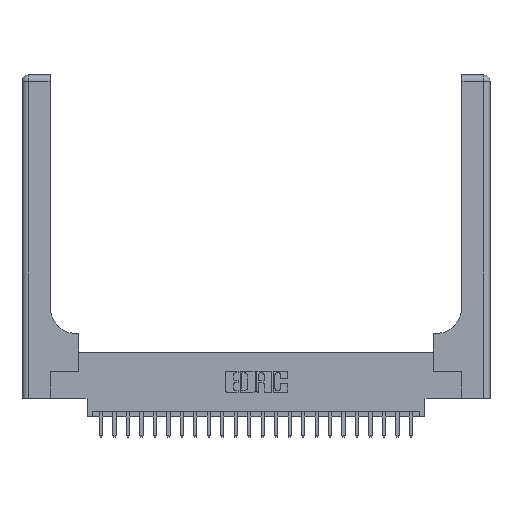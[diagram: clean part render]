
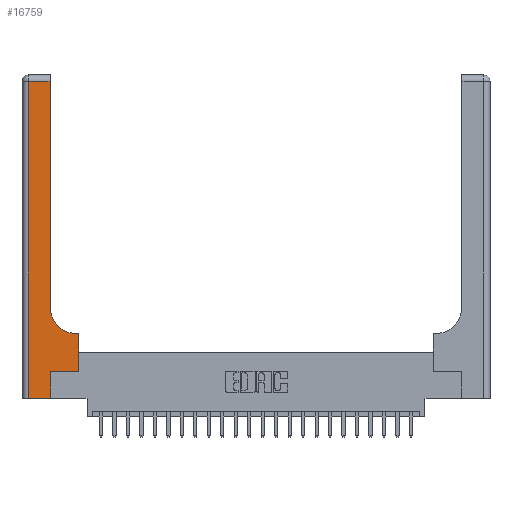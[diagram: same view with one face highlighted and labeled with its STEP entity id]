
A CAD part, top view. The second image highlights one B-rep face of the part: STEP entity #16759.
In plain terms, the highlighted planar face has unit normal (0, 0, 1).
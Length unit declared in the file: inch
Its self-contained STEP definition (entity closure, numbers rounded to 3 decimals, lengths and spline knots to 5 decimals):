
#467 = CARTESIAN_POINT ( 'NONE',  ( 0., 2.94, 0.37 ) ) ;
#500 = LINE ( 'NONE', #467, #5388 ) ;
#622 = ORIENTED_EDGE ( 'NONE', *, *, #14773, .T. ) ;
#769 = ORIENTED_EDGE ( 'NONE', *, *, #4746, .T. ) ;
#818 = EDGE_CURVE ( 'NONE', #1839, #12456, #20458, .T. ) ;
#1067 = ORIENTED_EDGE ( 'NONE', *, *, #16977, .T. ) ;
#1117 = AXIS2_PLACEMENT_3D ( 'NONE', #13332, #2342, #15140 ) ;
#1308 = ORIENTED_EDGE ( 'NONE', *, *, #20596, .T. ) ;
#1333 = CIRCLE ( 'NONE', #12049, 0.25 ) ;
#1466 = VERTEX_POINT ( 'NONE', #3202 ) ;
#1839 = VERTEX_POINT ( 'NONE', #16071 ) ;
#2086 = VERTEX_POINT ( 'NONE', #6284 ) ;
#2342 = DIRECTION ( 'NONE',  ( 0., 0., -1. ) ) ;
#2741 = CARTESIAN_POINT ( 'NONE',  ( 0.265, 0.25, 0.37 ) ) ;
#3039 = DIRECTION ( 'NONE',  ( -1., 0., 0. ) ) ;
#3202 = CARTESIAN_POINT ( 'NONE',  ( 0.26, 2.94, 0.37 ) ) ;
#3230 = EDGE_CURVE ( 'NONE', #19356, #1466, #9564, .T. ) ;
#4069 = VECTOR ( 'NONE', #13225, 39.37008 ) ;
#4310 = EDGE_CURVE ( 'NONE', #14408, #1839, #9453, .T. ) ;
#4746 = EDGE_CURVE ( 'NONE', #2086, #14117, #14071, .T. ) ;
#4954 = CARTESIAN_POINT ( 'NONE',  ( 0.26, 0.6, 0.37 ) ) ;
#5369 = ORIENTED_EDGE ( 'NONE', *, *, #3230, .T. ) ;
#5388 = VECTOR ( 'NONE', #11309, 39.37008 ) ;
#5515 = ORIENTED_EDGE ( 'NONE', *, *, #13615, .T. ) ;
#5915 = CARTESIAN_POINT ( 'NONE',  ( 0.26, 0.85, 0.37 ) ) ;
#6284 = CARTESIAN_POINT ( 'NONE',  ( 0.528, 0.25, 0.37 ) ) ;
#6522 = VECTOR ( 'NONE', #14974, 39.37008 ) ;
#7276 = LINE ( 'NONE', #4954, #16420 ) ;
#7803 = DIRECTION ( 'NONE',  ( 0., 0., -1. ) ) ;
#8040 = ORIENTED_EDGE ( 'NONE', *, *, #4310, .T. ) ;
#8920 = LINE ( 'NONE', #9505, #4069 ) ;
#9183 = VECTOR ( 'NONE', #17387, 39.37008 ) ;
#9430 = DIRECTION ( 'NONE',  ( 0., 1., 0. ) ) ;
#9453 = LINE ( 'NONE', #10834, #15457 ) ;
#9505 = CARTESIAN_POINT ( 'NONE',  ( 0.265, 0., 0.37 ) ) ;
#9511 = CARTESIAN_POINT ( 'NONE',  ( 0.26, 3., 0.37 ) ) ;
#9564 = LINE ( 'NONE', #9511, #18655 ) ;
#9961 = VERTEX_POINT ( 'NONE', #2741 ) ;
#10033 = CARTESIAN_POINT ( 'NONE',  ( 0.265, 0.25, 0.37 ) ) ;
#10834 = CARTESIAN_POINT ( 'NONE',  ( 0.06, 3., 0.37 ) ) ;
#10855 = VERTEX_POINT ( 'NONE', #13655 ) ;
#11309 = DIRECTION ( 'NONE',  ( -1., 0., 0. ) ) ;
#11474 = PLANE ( 'NONE',  #1117 ) ;
#11493 = CARTESIAN_POINT ( 'NONE',  ( 0.265, 0., 0.37 ) ) ;
#12049 = AXIS2_PLACEMENT_3D ( 'NONE', #18687, #7803, #20493 ) ;
#12456 = VERTEX_POINT ( 'NONE', #11493 ) ;
#13225 = DIRECTION ( 'NONE',  ( 0., 1., 0. ) ) ;
#13332 = CARTESIAN_POINT ( 'NONE',  ( 0., 3., 0.37 ) ) ;
#13438 = ORIENTED_EDGE ( 'NONE', *, *, #818, .T. ) ;
#13615 = EDGE_CURVE ( 'NONE', #1466, #14408, #500, .T. ) ;
#13655 = CARTESIAN_POINT ( 'NONE',  ( 0.51, 0.6, 0.37 ) ) ;
#14071 = LINE ( 'NONE', #19199, #9183 ) ;
#14117 = VERTEX_POINT ( 'NONE', #22760 ) ;
#14408 = VERTEX_POINT ( 'NONE', #18147 ) ;
#14773 = EDGE_CURVE ( 'NONE', #9961, #2086, #20445, .T. ) ;
#14955 = CARTESIAN_POINT ( 'NONE',  ( 0., 0., 0.37 ) ) ;
#14974 = DIRECTION ( 'NONE',  ( 1., 0., 0. ) ) ;
#15140 = DIRECTION ( 'NONE',  ( -1., 0., 0. ) ) ;
#15457 = VECTOR ( 'NONE', #23418, 39.37008 ) ;
#15565 = FACE_OUTER_BOUND ( 'NONE', #23441, .T. ) ;
#16007 = ORIENTED_EDGE ( 'NONE', *, *, #17323, .T. ) ;
#16071 = CARTESIAN_POINT ( 'NONE',  ( 0.06, 0., 0.37 ) ) ;
#16241 = VECTOR ( 'NONE', #22659, 39.37008 ) ;
#16420 = VECTOR ( 'NONE', #3039, 39.37008 ) ;
#16759 = ADVANCED_FACE ( 'NONE', ( #15565 ), #11474, .F. ) ;
#16977 = EDGE_CURVE ( 'NONE', #14117, #10855, #7276, .T. ) ;
#17323 = EDGE_CURVE ( 'NONE', #12456, #9961, #8920, .T. ) ;
#17387 = DIRECTION ( 'NONE',  ( 0., 1., 0. ) ) ;
#18147 = CARTESIAN_POINT ( 'NONE',  ( 0.06, 2.94, 0.37 ) ) ;
#18655 = VECTOR ( 'NONE', #9430, 39.37008 ) ;
#18687 = CARTESIAN_POINT ( 'NONE',  ( 0.51, 0.85, 0.37 ) ) ;
#19199 = CARTESIAN_POINT ( 'NONE',  ( 0.528, 0.25, 0.37 ) ) ;
#19356 = VERTEX_POINT ( 'NONE', #5915 ) ;
#20445 = LINE ( 'NONE', #10033, #16241 ) ;
#20458 = LINE ( 'NONE', #14955, #6522 ) ;
#20493 = DIRECTION ( 'NONE',  ( 1., 0., 0. ) ) ;
#20596 = EDGE_CURVE ( 'NONE', #10855, #19356, #1333, .T. ) ;
#22659 = DIRECTION ( 'NONE',  ( 1., 0., 0. ) ) ;
#22760 = CARTESIAN_POINT ( 'NONE',  ( 0.528, 0.6, 0.37 ) ) ;
#23418 = DIRECTION ( 'NONE',  ( 0., -1., 0. ) ) ;
#23441 = EDGE_LOOP ( 'NONE', ( #5369, #5515, #8040, #13438, #16007, #622, #769, #1067, #1308 ) ) ;
